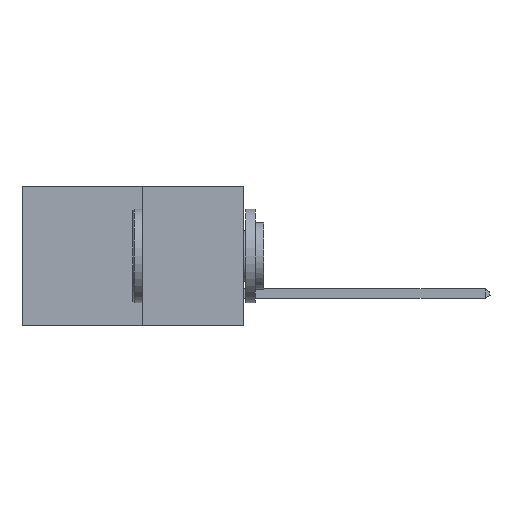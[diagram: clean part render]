
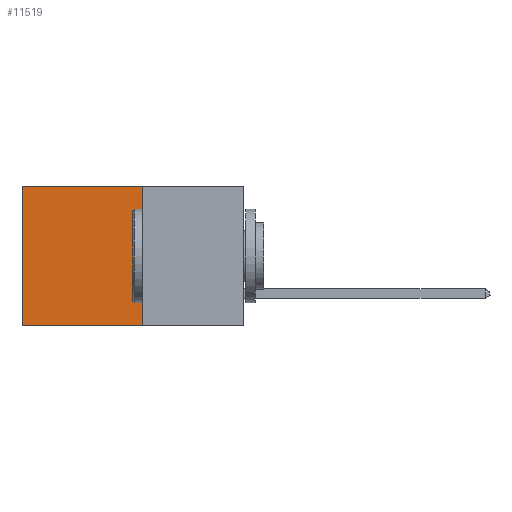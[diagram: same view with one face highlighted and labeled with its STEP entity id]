
A CAD part, left-side view. The second image highlights one B-rep face of the part: STEP entity #11519.
In plain terms, the highlighted planar face has unit normal (-1, 0, 0).
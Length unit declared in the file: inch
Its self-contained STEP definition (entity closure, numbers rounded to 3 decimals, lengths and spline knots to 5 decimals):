
#54 = EDGE_CURVE ( 'NONE', #14484, #882, #16788, .T. ) ;
#240 = EDGE_LOOP ( 'NONE', ( #11327, #14393, #5207, #10704 ) ) ;
#281 = VECTOR ( 'NONE', #5307, 39.37008 ) ;
#882 = VERTEX_POINT ( 'NONE', #4876 ) ;
#1121 = VECTOR ( 'NONE', #4169, 39.37008 ) ;
#2272 = PLANE ( 'NONE',  #13995 ) ;
#2480 = EDGE_CURVE ( 'NONE', #4735, #6563, #18945, .T. ) ;
#2992 = VECTOR ( 'NONE', #15695, 39.37008 ) ;
#3459 = LINE ( 'NONE', #15798, #13885 ) ;
#3803 = CARTESIAN_POINT ( 'NONE',  ( 0.277, 0.27, -0.37 ) ) ;
#3834 = DIRECTION ( 'NONE',  ( 0., 0., -1. ) ) ;
#4169 = DIRECTION ( 'NONE',  ( 0., 1., 0. ) ) ;
#4309 = LINE ( 'NONE', #3803, #281 ) ;
#4697 = CARTESIAN_POINT ( 'NONE',  ( 0.277, 0.27, 0. ) ) ;
#4735 = VERTEX_POINT ( 'NONE', #4774 ) ;
#4774 = CARTESIAN_POINT ( 'NONE',  ( 0.277, 0.27, -0.37 ) ) ;
#4876 = CARTESIAN_POINT ( 'NONE',  ( 0.277, 0.59, 0. ) ) ;
#5207 = ORIENTED_EDGE ( 'NONE', *, *, #13018, .F. ) ;
#5307 = DIRECTION ( 'NONE',  ( 0., 0., -1. ) ) ;
#5519 = CARTESIAN_POINT ( 'NONE',  ( 0.277, 0.27, 0. ) ) ;
#6563 = VERTEX_POINT ( 'NONE', #17947 ) ;
#8035 = EDGE_CURVE ( 'NONE', #882, #6563, #3459, .T. ) ;
#8227 = CARTESIAN_POINT ( 'NONE',  ( 0.277, 0.27, -0.37 ) ) ;
#10031 = DIRECTION ( 'NONE',  ( 0., 0., -1. ) ) ;
#10704 = ORIENTED_EDGE ( 'NONE', *, *, #54, .T. ) ;
#11327 = ORIENTED_EDGE ( 'NONE', *, *, #8035, .T. ) ;
#11519 = ADVANCED_FACE ( 'NONE', ( #12016 ), #2272, .F. ) ;
#12016 = FACE_OUTER_BOUND ( 'NONE', #240, .T. ) ;
#12467 = CARTESIAN_POINT ( 'NONE',  ( 0.277, 0.27, -0.37 ) ) ;
#12702 = DIRECTION ( 'NONE',  ( 1., 0., 0. ) ) ;
#13018 = EDGE_CURVE ( 'NONE', #14484, #4735, #4309, .T. ) ;
#13885 = VECTOR ( 'NONE', #10031, 39.37008 ) ;
#13995 = AXIS2_PLACEMENT_3D ( 'NONE', #8227, #12702, #3834 ) ;
#14393 = ORIENTED_EDGE ( 'NONE', *, *, #2480, .F. ) ;
#14484 = VERTEX_POINT ( 'NONE', #5519 ) ;
#15695 = DIRECTION ( 'NONE',  ( 0., 1., 0. ) ) ;
#15798 = CARTESIAN_POINT ( 'NONE',  ( 0.277, 0.59, -0.37 ) ) ;
#16788 = LINE ( 'NONE', #4697, #1121 ) ;
#17947 = CARTESIAN_POINT ( 'NONE',  ( 0.277, 0.59, -0.37 ) ) ;
#18945 = LINE ( 'NONE', #12467, #2992 ) ;
